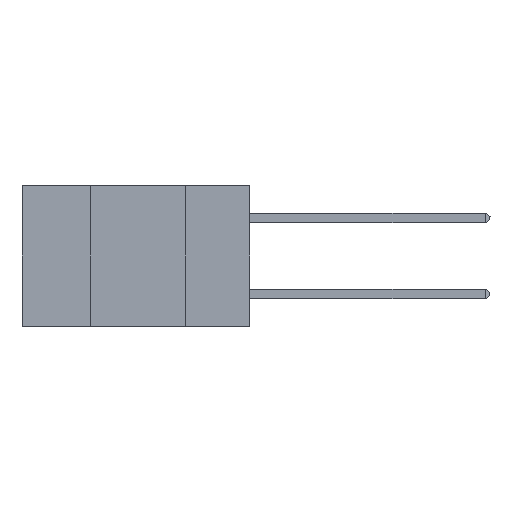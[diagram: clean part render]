
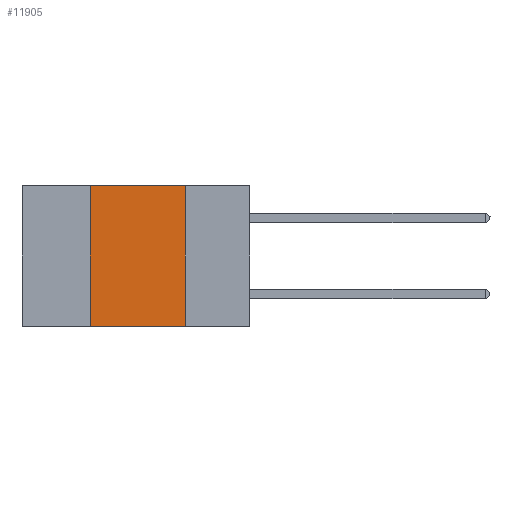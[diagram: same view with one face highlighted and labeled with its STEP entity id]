
A CAD part, left-side view. The second image highlights one B-rep face of the part: STEP entity #11905.
In plain terms, the highlighted planar face has unit normal (-1, 0, 0).
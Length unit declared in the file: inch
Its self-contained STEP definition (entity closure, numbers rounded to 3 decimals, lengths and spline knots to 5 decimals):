
#1768 = EDGE_LOOP ( 'NONE', ( #30296, #5892, #26942, #9841 ) ) ;
#2271 = PLANE ( 'NONE',  #21289 ) ;
#3822 = CARTESIAN_POINT ( 'NONE',  ( 0., 0.6, 0. ) ) ;
#4226 = DIRECTION ( 'NONE',  ( 0., 0., 1. ) ) ;
#4640 = LINE ( 'NONE', #37223, #8919 ) ;
#5892 = ORIENTED_EDGE ( 'NONE', *, *, #29030, .F. ) ;
#7703 = LINE ( 'NONE', #3822, #21009 ) ;
#7795 = FACE_OUTER_BOUND ( 'NONE', #1768, .T. ) ;
#8179 = VERTEX_POINT ( 'NONE', #25824 ) ;
#8919 = VECTOR ( 'NONE', #43534, 39.37008 ) ;
#9093 = DIRECTION ( 'NONE',  ( 1., 0., 0. ) ) ;
#9841 = ORIENTED_EDGE ( 'NONE', *, *, #37715, .T. ) ;
#11014 = LINE ( 'NONE', #26754, #38752 ) ;
#11905 = ADVANCED_FACE ( 'NONE', ( #7795 ), #2271, .F. ) ;
#12516 = DIRECTION ( 'NONE',  ( 0., 0., -1. ) ) ;
#14156 = CARTESIAN_POINT ( 'NONE',  ( 0., 0.42, 0. ) ) ;
#15678 = VERTEX_POINT ( 'NONE', #42375 ) ;
#19631 = DIRECTION ( 'NONE',  ( 0., 0., -1. ) ) ;
#21009 = VECTOR ( 'NONE', #42700, 39.37008 ) ;
#21289 = AXIS2_PLACEMENT_3D ( 'NONE', #26021, #9093, #12516 ) ;
#23239 = CARTESIAN_POINT ( 'NONE',  ( 0., 0.17, -0.37 ) ) ;
#25382 = VECTOR ( 'NONE', #4226, 39.37008 ) ;
#25824 = CARTESIAN_POINT ( 'NONE',  ( 0., 0.17, 0. ) ) ;
#26021 = CARTESIAN_POINT ( 'NONE',  ( 0., 0.6, 0. ) ) ;
#26214 = EDGE_CURVE ( 'NONE', #15678, #36056, #32295, .T. ) ;
#26754 = CARTESIAN_POINT ( 'NONE',  ( 0., 0.17, 0. ) ) ;
#26942 = ORIENTED_EDGE ( 'NONE', *, *, #26214, .F. ) ;
#29030 = EDGE_CURVE ( 'NONE', #36056, #8179, #7703, .T. ) ;
#29439 = CARTESIAN_POINT ( 'NONE',  ( 0., 0.42, 0. ) ) ;
#30296 = ORIENTED_EDGE ( 'NONE', *, *, #34011, .F. ) ;
#32295 = LINE ( 'NONE', #14156, #25382 ) ;
#34011 = EDGE_CURVE ( 'NONE', #8179, #37792, #11014, .T. ) ;
#36056 = VERTEX_POINT ( 'NONE', #29439 ) ;
#37223 = CARTESIAN_POINT ( 'NONE',  ( 0., 0.6, -0.37 ) ) ;
#37715 = EDGE_CURVE ( 'NONE', #15678, #37792, #4640, .T. ) ;
#37792 = VERTEX_POINT ( 'NONE', #23239 ) ;
#38752 = VECTOR ( 'NONE', #19631, 39.37008 ) ;
#42375 = CARTESIAN_POINT ( 'NONE',  ( 0., 0.42, -0.37 ) ) ;
#42700 = DIRECTION ( 'NONE',  ( 0., -1., 0. ) ) ;
#43534 = DIRECTION ( 'NONE',  ( 0., -1., 0. ) ) ;
